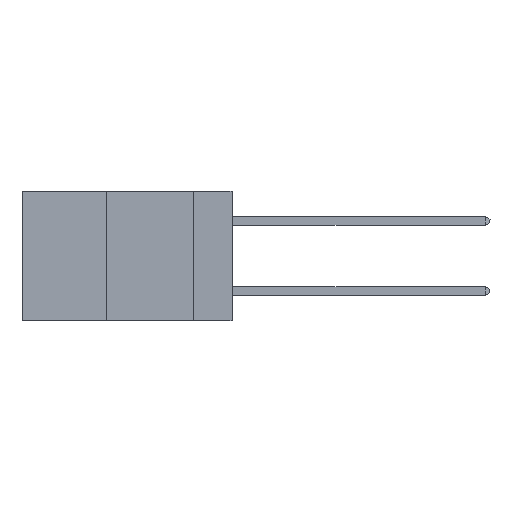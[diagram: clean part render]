
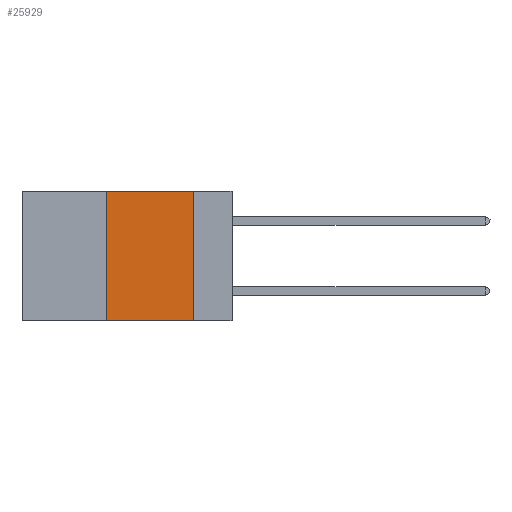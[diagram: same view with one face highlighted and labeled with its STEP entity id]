
A CAD part, left-side view. The second image highlights one B-rep face of the part: STEP entity #25929.
In plain terms, the highlighted planar face has unit normal (-1, 0, 0).
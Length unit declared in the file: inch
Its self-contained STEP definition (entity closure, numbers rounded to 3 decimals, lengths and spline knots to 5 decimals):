
#864 = ORIENTED_EDGE ( 'NONE', *, *, #16756, .F. ) ;
#3442 = FACE_OUTER_BOUND ( 'NONE', #17251, .T. ) ;
#6007 = DIRECTION ( 'NONE',  ( 0., 0., 1. ) ) ;
#7448 = CARTESIAN_POINT ( 'NONE',  ( 0., 0.11, -0.37 ) ) ;
#8505 = ORIENTED_EDGE ( 'NONE', *, *, #15128, .F. ) ;
#10085 = VECTOR ( 'NONE', #31137, 39.37008 ) ;
#10094 = VECTOR ( 'NONE', #6007, 39.37008 ) ;
#10441 = VECTOR ( 'NONE', #34050, 39.37008 ) ;
#12849 = VERTEX_POINT ( 'NONE', #39944 ) ;
#13459 = CARTESIAN_POINT ( 'NONE',  ( 0., 0.6, -0.37 ) ) ;
#15128 = EDGE_CURVE ( 'NONE', #15715, #19969, #39316, .T. ) ;
#15715 = VERTEX_POINT ( 'NONE', #37190 ) ;
#15756 = CARTESIAN_POINT ( 'NONE',  ( 0., 0.11, 0. ) ) ;
#16756 = EDGE_CURVE ( 'NONE', #12849, #15715, #39652, .T. ) ;
#17160 = CARTESIAN_POINT ( 'NONE',  ( 0., 0.6, 0. ) ) ;
#17251 = EDGE_LOOP ( 'NONE', ( #30284, #8505, #864, #22733 ) ) ;
#17569 = DIRECTION ( 'NONE',  ( 0., -1., 0. ) ) ;
#18518 = VECTOR ( 'NONE', #17569, 39.37008 ) ;
#19242 = EDGE_CURVE ( 'NONE', #19969, #22353, #31938, .T. ) ;
#19426 = DIRECTION ( 'NONE',  ( 0., 0., -1. ) ) ;
#19969 = VERTEX_POINT ( 'NONE', #36598 ) ;
#21905 = CARTESIAN_POINT ( 'NONE',  ( 0., 0.6, 0. ) ) ;
#22353 = VERTEX_POINT ( 'NONE', #7448 ) ;
#22733 = ORIENTED_EDGE ( 'NONE', *, *, #39179, .T. ) ;
#25381 = DIRECTION ( 'NONE',  ( 1., 0., 0. ) ) ;
#25929 = ADVANCED_FACE ( 'NONE', ( #3442 ), #34623, .F. ) ;
#29964 = AXIS2_PLACEMENT_3D ( 'NONE', #21905, #25381, #19426 ) ;
#30284 = ORIENTED_EDGE ( 'NONE', *, *, #19242, .F. ) ;
#31137 = DIRECTION ( 'NONE',  ( 0., 0., -1. ) ) ;
#31372 = LINE ( 'NONE', #13459, #10441 ) ;
#31938 = LINE ( 'NONE', #15756, #10085 ) ;
#34050 = DIRECTION ( 'NONE',  ( 0., -1., 0. ) ) ;
#34623 = PLANE ( 'NONE',  #29964 ) ;
#36598 = CARTESIAN_POINT ( 'NONE',  ( 0., 0.11, 0. ) ) ;
#37190 = CARTESIAN_POINT ( 'NONE',  ( 0., 0.36, 0. ) ) ;
#39179 = EDGE_CURVE ( 'NONE', #12849, #22353, #31372, .T. ) ;
#39316 = LINE ( 'NONE', #17160, #18518 ) ;
#39652 = LINE ( 'NONE', #40062, #10094 ) ;
#39944 = CARTESIAN_POINT ( 'NONE',  ( 0., 0.36, -0.37 ) ) ;
#40062 = CARTESIAN_POINT ( 'NONE',  ( 0., 0.36, 0. ) ) ;
